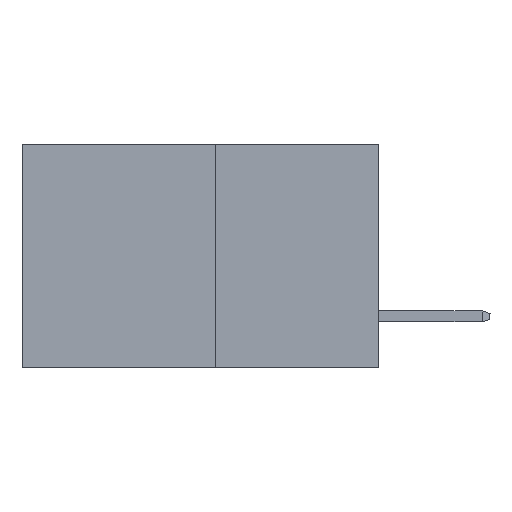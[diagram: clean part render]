
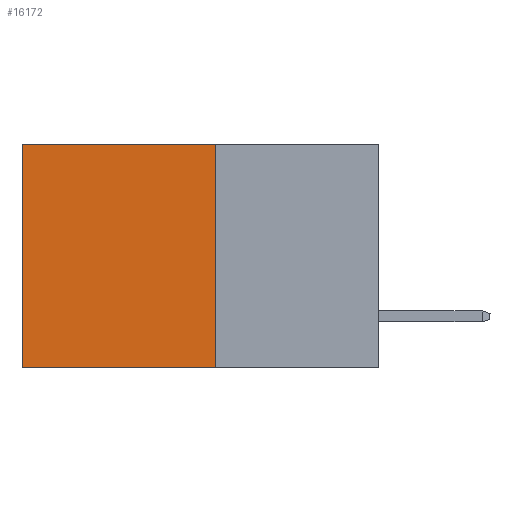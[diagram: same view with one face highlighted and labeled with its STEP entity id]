
A CAD part, left-side view. The second image highlights one B-rep face of the part: STEP entity #16172.
In plain terms, the highlighted planar face has unit normal (-1, 0, 0).
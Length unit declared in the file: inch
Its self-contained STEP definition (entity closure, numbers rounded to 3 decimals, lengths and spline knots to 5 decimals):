
#1150 = EDGE_LOOP ( 'NONE', ( #21288, #4899, #23480, #14600 ) ) ;
#1993 = DIRECTION ( 'NONE',  ( 0., 1., 0. ) ) ;
#2197 = CARTESIAN_POINT ( 'NONE',  ( 0.277, 0.59, 0. ) ) ;
#2234 = LINE ( 'NONE', #7909, #26393 ) ;
#4899 = ORIENTED_EDGE ( 'NONE', *, *, #16398, .F. ) ;
#5680 = EDGE_CURVE ( 'NONE', #9837, #6282, #28859, .T. ) ;
#5711 = CARTESIAN_POINT ( 'NONE',  ( 0.277, 0.27, -0.37 ) ) ;
#5834 = DIRECTION ( 'NONE',  ( 0., 1., 0. ) ) ;
#6241 = CARTESIAN_POINT ( 'NONE',  ( 0.277, 0.27, -0.37 ) ) ;
#6282 = VERTEX_POINT ( 'NONE', #2197 ) ;
#7909 = CARTESIAN_POINT ( 'NONE',  ( 0.277, 0.59, -0.37 ) ) ;
#8529 = DIRECTION ( 'NONE',  ( 0., 0., -1. ) ) ;
#9837 = VERTEX_POINT ( 'NONE', #16446 ) ;
#10246 = DIRECTION ( 'NONE',  ( 0., 0., -1. ) ) ;
#11866 = EDGE_CURVE ( 'NONE', #6282, #16987, #2234, .T. ) ;
#12660 = LINE ( 'NONE', #6241, #23831 ) ;
#13191 = CARTESIAN_POINT ( 'NONE',  ( 0.277, 0.27, -0.37 ) ) ;
#14600 = ORIENTED_EDGE ( 'NONE', *, *, #5680, .T. ) ;
#15248 = AXIS2_PLACEMENT_3D ( 'NONE', #5711, #23648, #10246 ) ;
#15780 = VERTEX_POINT ( 'NONE', #16044 ) ;
#16044 = CARTESIAN_POINT ( 'NONE',  ( 0.277, 0.27, -0.37 ) ) ;
#16172 = ADVANCED_FACE ( 'NONE', ( #25291 ), #21398, .F. ) ;
#16398 = EDGE_CURVE ( 'NONE', #15780, #16987, #20372, .T. ) ;
#16446 = CARTESIAN_POINT ( 'NONE',  ( 0.277, 0.27, 0. ) ) ;
#16638 = CARTESIAN_POINT ( 'NONE',  ( 0.277, 0.27, 0. ) ) ;
#16987 = VERTEX_POINT ( 'NONE', #17160 ) ;
#17068 = EDGE_CURVE ( 'NONE', #9837, #15780, #12660, .T. ) ;
#17160 = CARTESIAN_POINT ( 'NONE',  ( 0.277, 0.59, -0.37 ) ) ;
#17660 = VECTOR ( 'NONE', #5834, 39.37008 ) ;
#19685 = VECTOR ( 'NONE', #1993, 39.37008 ) ;
#20372 = LINE ( 'NONE', #13191, #19685 ) ;
#21288 = ORIENTED_EDGE ( 'NONE', *, *, #11866, .T. ) ;
#21398 = PLANE ( 'NONE',  #15248 ) ;
#23480 = ORIENTED_EDGE ( 'NONE', *, *, #17068, .F. ) ;
#23648 = DIRECTION ( 'NONE',  ( 1., 0., 0. ) ) ;
#23831 = VECTOR ( 'NONE', #8529, 39.37008 ) ;
#25291 = FACE_OUTER_BOUND ( 'NONE', #1150, .T. ) ;
#26393 = VECTOR ( 'NONE', #26755, 39.37008 ) ;
#26755 = DIRECTION ( 'NONE',  ( 0., 0., -1. ) ) ;
#28859 = LINE ( 'NONE', #16638, #17660 ) ;
